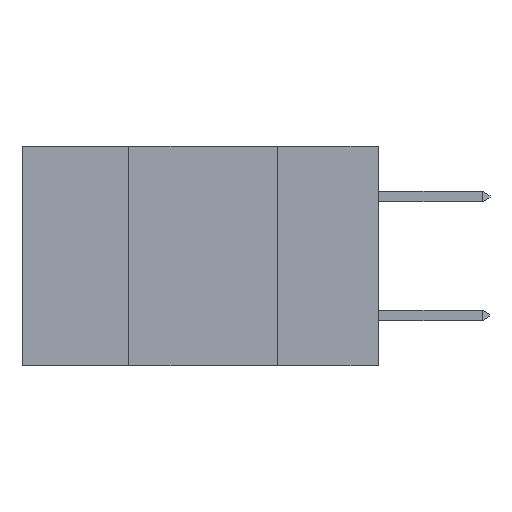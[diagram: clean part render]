
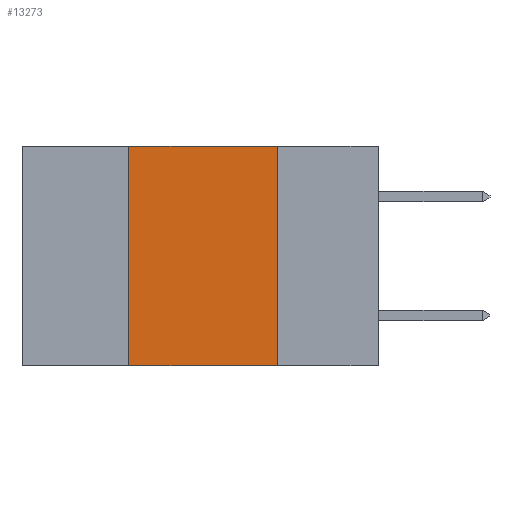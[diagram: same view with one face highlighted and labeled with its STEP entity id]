
A CAD part, left-side view. The second image highlights one B-rep face of the part: STEP entity #13273.
In plain terms, the highlighted planar face has unit normal (-1, 0, 0).
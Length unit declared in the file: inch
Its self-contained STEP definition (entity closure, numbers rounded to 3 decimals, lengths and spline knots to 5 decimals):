
#61 = DIRECTION ( 'NONE',  ( 0., -1., 0. ) ) ;
#642 = CARTESIAN_POINT ( 'NONE',  ( 0., 0.6, 0. ) ) ;
#2439 = EDGE_CURVE ( 'NONE', #9291, #10089, #9785, .T. ) ;
#2519 = EDGE_LOOP ( 'NONE', ( #5633, #20973, #18436, #9220 ) ) ;
#2797 = AXIS2_PLACEMENT_3D ( 'NONE', #15750, #4750, #17556 ) ;
#3879 = DIRECTION ( 'NONE',  ( 0., 0., -1. ) ) ;
#4048 = VECTOR ( 'NONE', #20818, 39.37008 ) ;
#4750 = DIRECTION ( 'NONE',  ( 1., 0., 0. ) ) ;
#5633 = ORIENTED_EDGE ( 'NONE', *, *, #22347, .F. ) ;
#7001 = VECTOR ( 'NONE', #14450, 39.37008 ) ;
#7048 = CARTESIAN_POINT ( 'NONE',  ( 0., 0.42, 0. ) ) ;
#7124 = CARTESIAN_POINT ( 'NONE',  ( 0., 0.17, -0.37 ) ) ;
#7369 = VERTEX_POINT ( 'NONE', #7124 ) ;
#7903 = VERTEX_POINT ( 'NONE', #17574 ) ;
#8463 = EDGE_CURVE ( 'NONE', #7903, #7369, #13867, .T. ) ;
#9220 = ORIENTED_EDGE ( 'NONE', *, *, #8463, .T. ) ;
#9291 = VERTEX_POINT ( 'NONE', #23441 ) ;
#9785 = LINE ( 'NONE', #642, #21380 ) ;
#9990 = CARTESIAN_POINT ( 'NONE',  ( 0., 0.6, -0.37 ) ) ;
#10089 = VERTEX_POINT ( 'NONE', #20045 ) ;
#10165 = PLANE ( 'NONE',  #2797 ) ;
#11906 = LINE ( 'NONE', #7048, #7001 ) ;
#13273 = ADVANCED_FACE ( 'NONE', ( #23437 ), #10165, .F. ) ;
#13867 = LINE ( 'NONE', #9990, #4048 ) ;
#14450 = DIRECTION ( 'NONE',  ( 0., 0., 1. ) ) ;
#15750 = CARTESIAN_POINT ( 'NONE',  ( 0., 0.6, 0. ) ) ;
#17556 = DIRECTION ( 'NONE',  ( 0., 0., -1. ) ) ;
#17574 = CARTESIAN_POINT ( 'NONE',  ( 0., 0.42, -0.37 ) ) ;
#18436 = ORIENTED_EDGE ( 'NONE', *, *, #22173, .F. ) ;
#20045 = CARTESIAN_POINT ( 'NONE',  ( 0., 0.17, 0. ) ) ;
#20818 = DIRECTION ( 'NONE',  ( 0., -1., 0. ) ) ;
#20973 = ORIENTED_EDGE ( 'NONE', *, *, #2439, .F. ) ;
#21380 = VECTOR ( 'NONE', #61, 39.37008 ) ;
#22064 = CARTESIAN_POINT ( 'NONE',  ( 0., 0.17, 0. ) ) ;
#22173 = EDGE_CURVE ( 'NONE', #7903, #9291, #11906, .T. ) ;
#22347 = EDGE_CURVE ( 'NONE', #10089, #7369, #22926, .T. ) ;
#22350 = VECTOR ( 'NONE', #3879, 39.37008 ) ;
#22926 = LINE ( 'NONE', #22064, #22350 ) ;
#23437 = FACE_OUTER_BOUND ( 'NONE', #2519, .T. ) ;
#23441 = CARTESIAN_POINT ( 'NONE',  ( 0., 0.42, 0. ) ) ;
